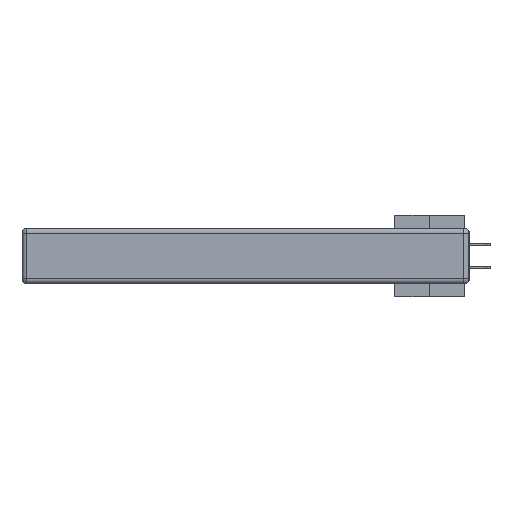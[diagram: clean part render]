
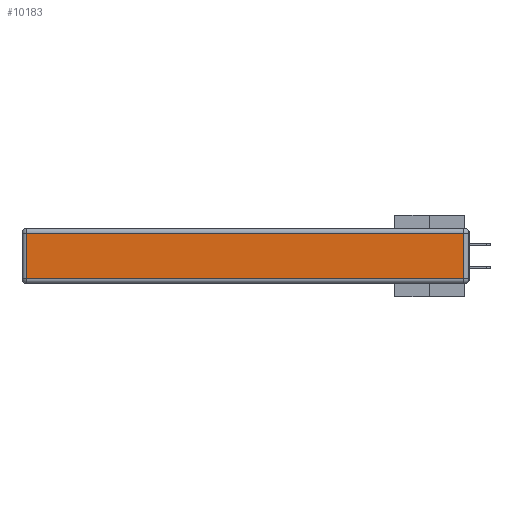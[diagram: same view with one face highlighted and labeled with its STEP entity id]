
A CAD part, left-side view. The second image highlights one B-rep face of the part: STEP entity #10183.
In plain terms, the highlighted planar face has unit normal (-1, 0, 0).
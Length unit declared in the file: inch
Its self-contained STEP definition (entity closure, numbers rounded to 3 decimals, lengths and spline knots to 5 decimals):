
#783 = CARTESIAN_POINT ( 'NONE',  ( 0., 2.75, -0.03 ) ) ;
#2969 = CARTESIAN_POINT ( 'NONE',  ( 0., 0.03, -0.313 ) ) ;
#3393 = DIRECTION ( 'NONE',  ( 0., -1., 0. ) ) ;
#3775 = DIRECTION ( 'NONE',  ( -1., 0., 0. ) ) ;
#4307 = CARTESIAN_POINT ( 'NONE',  ( 0., 0.03, -0.03 ) ) ;
#5640 = EDGE_CURVE ( 'NONE', #7634, #24130, #36451, .T. ) ;
#5759 = ORIENTED_EDGE ( 'NONE', *, *, #10069, .T. ) ;
#5870 = DIRECTION ( 'NONE',  ( 0., 0., 1. ) ) ;
#7634 = VERTEX_POINT ( 'NONE', #4307 ) ;
#8177 = VECTOR ( 'NONE', #20552, 39.37008 ) ;
#8292 = FACE_OUTER_BOUND ( 'NONE', #35540, .T. ) ;
#9228 = CARTESIAN_POINT ( 'NONE',  ( 0., 0., -0.313 ) ) ;
#9685 = LINE ( 'NONE', #30202, #10552 ) ;
#10069 = EDGE_CURVE ( 'NONE', #20750, #34551, #24639, .T. ) ;
#10183 = ADVANCED_FACE ( 'NONE', ( #8292 ), #29210, .T. ) ;
#10552 = VECTOR ( 'NONE', #26866, 39.37008 ) ;
#12117 = ORIENTED_EDGE ( 'NONE', *, *, #14632, .T. ) ;
#14632 = EDGE_CURVE ( 'NONE', #24130, #20750, #9685, .T. ) ;
#15369 = CARTESIAN_POINT ( 'NONE',  ( 0., 0., -0.343 ) ) ;
#17585 = AXIS2_PLACEMENT_3D ( 'NONE', #15369, #3775, #35239 ) ;
#17606 = VECTOR ( 'NONE', #3393, 39.37008 ) ;
#18272 = EDGE_CURVE ( 'NONE', #34551, #7634, #29848, .T. ) ;
#20200 = CARTESIAN_POINT ( 'NONE',  ( 0., 2.72, -0.03 ) ) ;
#20552 = DIRECTION ( 'NONE',  ( 0., 1., 0. ) ) ;
#20750 = VERTEX_POINT ( 'NONE', #30824 ) ;
#24130 = VERTEX_POINT ( 'NONE', #20200 ) ;
#24639 = LINE ( 'NONE', #9228, #17606 ) ;
#25752 = ORIENTED_EDGE ( 'NONE', *, *, #18272, .T. ) ;
#26716 = VECTOR ( 'NONE', #5870, 39.37008 ) ;
#26866 = DIRECTION ( 'NONE',  ( 0., 0., -1. ) ) ;
#29210 = PLANE ( 'NONE',  #17585 ) ;
#29848 = LINE ( 'NONE', #31070, #26716 ) ;
#30202 = CARTESIAN_POINT ( 'NONE',  ( 0., 2.72, -0.343 ) ) ;
#30824 = CARTESIAN_POINT ( 'NONE',  ( 0., 2.72, -0.313 ) ) ;
#31070 = CARTESIAN_POINT ( 'NONE',  ( 0., 0.03, -0.343 ) ) ;
#32854 = ORIENTED_EDGE ( 'NONE', *, *, #5640, .T. ) ;
#34551 = VERTEX_POINT ( 'NONE', #2969 ) ;
#35239 = DIRECTION ( 'NONE',  ( 0., 0., 1. ) ) ;
#35540 = EDGE_LOOP ( 'NONE', ( #5759, #25752, #32854, #12117 ) ) ;
#36451 = LINE ( 'NONE', #783, #8177 ) ;
